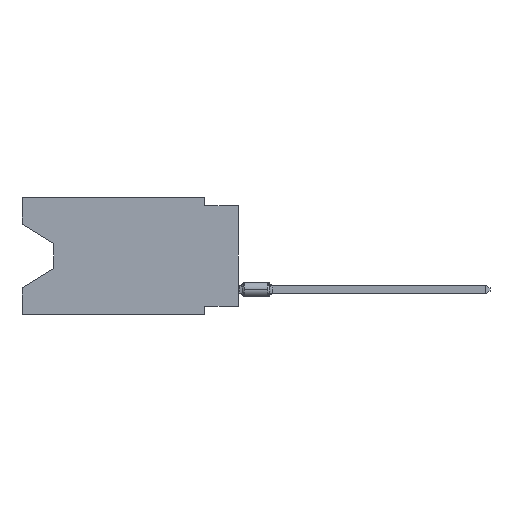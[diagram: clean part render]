
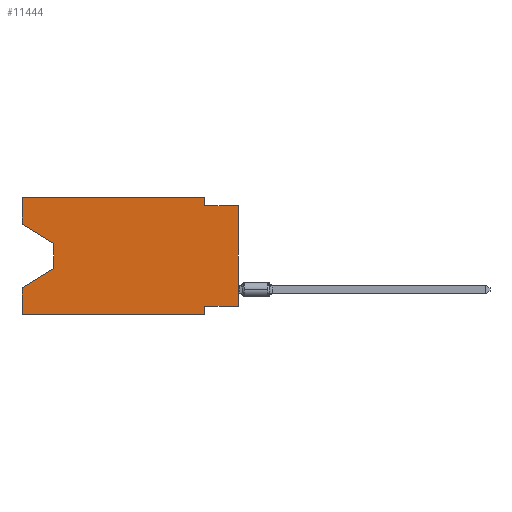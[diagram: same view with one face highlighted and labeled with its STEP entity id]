
A CAD part, left-side view. The second image highlights one B-rep face of the part: STEP entity #11444.
In plain terms, the highlighted planar face has unit normal (-1, 0, 0).
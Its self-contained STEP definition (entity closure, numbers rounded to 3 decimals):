
#235 = EDGE_CURVE ( 'NONE', #17926, #20014, #3368, .T. ) ;
#254 = LINE ( 'NONE', #7653, #21075 ) ;
#687 = EDGE_CURVE ( 'NONE', #2582, #11586, #19929, .T. ) ;
#700 = CARTESIAN_POINT ( 'NONE',  ( 0., 2.54, -0.635 ) ) ;
#869 = DIRECTION ( 'NONE',  ( 0., 0., 1. ) ) ;
#872 = EDGE_CURVE ( 'NONE', #9316, #19171, #11452, .T. ) ;
#884 = CARTESIAN_POINT ( 'NONE',  ( 0., 16.383, 0. ) ) ;
#1448 = EDGE_CURVE ( 'NONE', #20586, #20245, #21103, .T. ) ;
#1515 = ORIENTED_EDGE ( 'NONE', *, *, #1448, .F. ) ;
#2170 = LINE ( 'NONE', #9558, #21520 ) ;
#2579 = AXIS2_PLACEMENT_3D ( 'NONE', #9636, #22351, #16521 ) ;
#2582 = VERTEX_POINT ( 'NONE', #7052 ) ;
#2761 = CARTESIAN_POINT ( 'NONE',  ( 0., 13.97, -5.385 ) ) ;
#2803 = CARTESIAN_POINT ( 'NONE',  ( 0., 16.383, -2.038 ) ) ;
#3009 = DIRECTION ( 'NONE',  ( 0., 0.855, -0.519 ) ) ;
#3368 = LINE ( 'NONE', #21546, #5911 ) ;
#3916 = CARTESIAN_POINT ( 'NONE',  ( 0., 16.383, -6.852 ) ) ;
#4170 = ORIENTED_EDGE ( 'NONE', *, *, #872, .F. ) ;
#4547 = DIRECTION ( 'NONE',  ( 0., 0., -1. ) ) ;
#5685 = DIRECTION ( 'NONE',  ( 0., -1., 0. ) ) ;
#5911 = VECTOR ( 'NONE', #10641, 1000. ) ;
#5959 = CARTESIAN_POINT ( 'NONE',  ( 0., 2.54, 0. ) ) ;
#6160 = CARTESIAN_POINT ( 'NONE',  ( 0., 2.54, -8.89 ) ) ;
#6183 = DIRECTION ( 'NONE',  ( 0., 0., 1. ) ) ;
#6225 = ORIENTED_EDGE ( 'NONE', *, *, #21187, .F. ) ;
#6300 = CARTESIAN_POINT ( 'NONE',  ( 0., 16.383, -2.038 ) ) ;
#6723 = CARTESIAN_POINT ( 'NONE',  ( 0., 2.54, -8.89 ) ) ;
#6822 = EDGE_LOOP ( 'NONE', ( #15934, #8828, #14101, #1515, #21080, #13259, #11789, #9339, #6225, #11917, #14948, #4170 ) ) ;
#7052 = CARTESIAN_POINT ( 'NONE',  ( 0., 13.97, -3.505 ) ) ;
#7220 = VECTOR ( 'NONE', #7349, 1000. ) ;
#7281 = EDGE_CURVE ( 'NONE', #20309, #17678, #11877, .T. ) ;
#7291 = CARTESIAN_POINT ( 'NONE',  ( 0., 16.383, -8.89 ) ) ;
#7349 = DIRECTION ( 'NONE',  ( 0., -1., 0. ) ) ;
#7653 = CARTESIAN_POINT ( 'NONE',  ( 0., 0., -8.255 ) ) ;
#7778 = LINE ( 'NONE', #6300, #23926 ) ;
#8777 = CARTESIAN_POINT ( 'NONE',  ( 0., 0., -0.635 ) ) ;
#8828 = ORIENTED_EDGE ( 'NONE', *, *, #687, .T. ) ;
#9089 = VECTOR ( 'NONE', #869, 1000. ) ;
#9316 = VERTEX_POINT ( 'NONE', #2803 ) ;
#9339 = ORIENTED_EDGE ( 'NONE', *, *, #7281, .T. ) ;
#9558 = CARTESIAN_POINT ( 'NONE',  ( 0., 0., -0.635 ) ) ;
#9636 = CARTESIAN_POINT ( 'NONE',  ( 0., 16.383, 0. ) ) ;
#10152 = VECTOR ( 'NONE', #6183, 1000. ) ;
#10641 = DIRECTION ( 'NONE',  ( 0., 0., -1. ) ) ;
#10663 = CARTESIAN_POINT ( 'NONE',  ( 0., 16.383, 0. ) ) ;
#11444 = ADVANCED_FACE ( 'NONE', ( #20531 ), #15176, .F. ) ;
#11452 = LINE ( 'NONE', #12889, #20675 ) ;
#11586 = VERTEX_POINT ( 'NONE', #19299 ) ;
#11789 = ORIENTED_EDGE ( 'NONE', *, *, #19548, .F. ) ;
#11877 = LINE ( 'NONE', #19483, #10152 ) ;
#11917 = ORIENTED_EDGE ( 'NONE', *, *, #235, .F. ) ;
#12545 = LINE ( 'NONE', #23933, #7220 ) ;
#12889 = CARTESIAN_POINT ( 'NONE',  ( 0., 16.383, 0. ) ) ;
#13259 = ORIENTED_EDGE ( 'NONE', *, *, #23189, .F. ) ;
#13513 = VERTEX_POINT ( 'NONE', #17155 ) ;
#14101 = ORIENTED_EDGE ( 'NONE', *, *, #22496, .T. ) ;
#14110 = DIRECTION ( 'NONE',  ( 0., 0., -1. ) ) ;
#14126 = VECTOR ( 'NONE', #3009, 1000. ) ;
#14150 = EDGE_CURVE ( 'NONE', #19171, #17926, #15290, .T. ) ;
#14609 = EDGE_CURVE ( 'NONE', #9316, #2582, #7778, .T. ) ;
#14948 = ORIENTED_EDGE ( 'NONE', *, *, #14150, .F. ) ;
#15017 = DIRECTION ( 'NONE',  ( 0., 1., 0. ) ) ;
#15176 = PLANE ( 'NONE',  #2579 ) ;
#15290 = LINE ( 'NONE', #884, #19277 ) ;
#15934 = ORIENTED_EDGE ( 'NONE', *, *, #14609, .T. ) ;
#16521 = DIRECTION ( 'NONE',  ( 0., 0., -1. ) ) ;
#17155 = CARTESIAN_POINT ( 'NONE',  ( 0., 2.54, -8.255 ) ) ;
#17218 = CARTESIAN_POINT ( 'NONE',  ( 0., 0., -8.255 ) ) ;
#17447 = CARTESIAN_POINT ( 'NONE',  ( 0., 16.383, 0. ) ) ;
#17678 = VERTEX_POINT ( 'NONE', #8777 ) ;
#17926 = VERTEX_POINT ( 'NONE', #5959 ) ;
#18468 = DIRECTION ( 'NONE',  ( 0., 0., 1. ) ) ;
#18830 = VECTOR ( 'NONE', #4547, 1000. ) ;
#18902 = DIRECTION ( 'NONE',  ( 0., -0.855, -0.519 ) ) ;
#19171 = VERTEX_POINT ( 'NONE', #10663 ) ;
#19277 = VECTOR ( 'NONE', #22932, 1000. ) ;
#19299 = CARTESIAN_POINT ( 'NONE',  ( 0., 13.97, -5.385 ) ) ;
#19483 = CARTESIAN_POINT ( 'NONE',  ( 0., 0., 0. ) ) ;
#19548 = EDGE_CURVE ( 'NONE', #20309, #13513, #254, .T. ) ;
#19574 = CARTESIAN_POINT ( 'NONE',  ( 0., 13.97, -3.505 ) ) ;
#19929 = LINE ( 'NONE', #19574, #22232 ) ;
#20014 = VERTEX_POINT ( 'NONE', #700 ) ;
#20245 = VERTEX_POINT ( 'NONE', #3916 ) ;
#20309 = VERTEX_POINT ( 'NONE', #17218 ) ;
#20531 = FACE_OUTER_BOUND ( 'NONE', #6822, .T. ) ;
#20586 = VERTEX_POINT ( 'NONE', #7291 ) ;
#20675 = VECTOR ( 'NONE', #18468, 1000. ) ;
#21075 = VECTOR ( 'NONE', #15017, 1000. ) ;
#21080 = ORIENTED_EDGE ( 'NONE', *, *, #21465, .T. ) ;
#21103 = LINE ( 'NONE', #17447, #9089 ) ;
#21149 = LINE ( 'NONE', #6723, #18830 ) ;
#21187 = EDGE_CURVE ( 'NONE', #20014, #17678, #2170, .T. ) ;
#21465 = EDGE_CURVE ( 'NONE', #20586, #22353, #12545, .T. ) ;
#21520 = VECTOR ( 'NONE', #5685, 1000. ) ;
#21546 = CARTESIAN_POINT ( 'NONE',  ( 0., 2.54, 0. ) ) ;
#22232 = VECTOR ( 'NONE', #14110, 1000. ) ;
#22351 = DIRECTION ( 'NONE',  ( 1., 0., 0. ) ) ;
#22353 = VERTEX_POINT ( 'NONE', #6160 ) ;
#22496 = EDGE_CURVE ( 'NONE', #11586, #20245, #22987, .T. ) ;
#22932 = DIRECTION ( 'NONE',  ( 0., -1., 0. ) ) ;
#22987 = LINE ( 'NONE', #2761, #14126 ) ;
#23189 = EDGE_CURVE ( 'NONE', #13513, #22353, #21149, .T. ) ;
#23926 = VECTOR ( 'NONE', #18902, 1000. ) ;
#23933 = CARTESIAN_POINT ( 'NONE',  ( 0., 16.383, -8.89 ) ) ;
